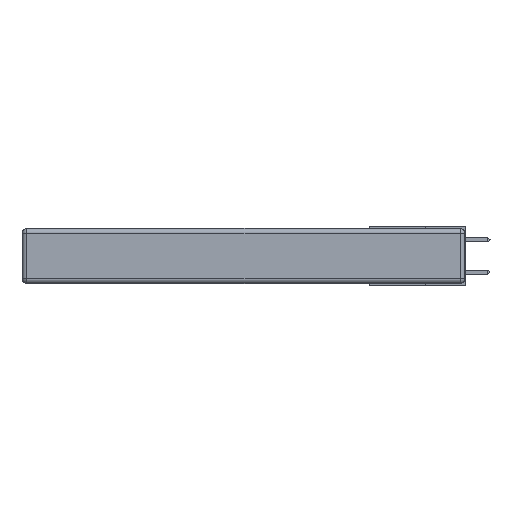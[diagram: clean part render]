
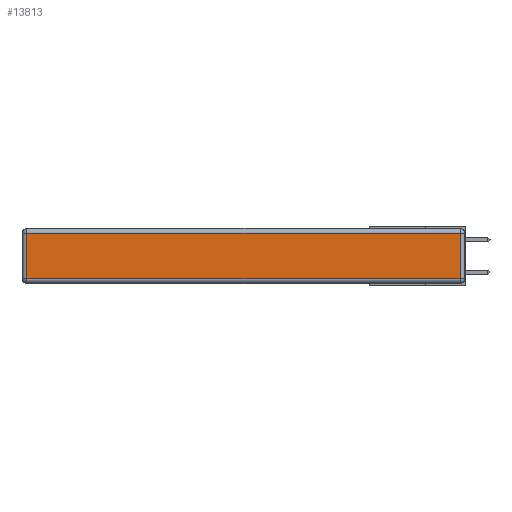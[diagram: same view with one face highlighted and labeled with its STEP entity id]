
A CAD part, left-side view. The second image highlights one B-rep face of the part: STEP entity #13813.
In plain terms, the highlighted planar face has unit normal (-1, 0, 0).
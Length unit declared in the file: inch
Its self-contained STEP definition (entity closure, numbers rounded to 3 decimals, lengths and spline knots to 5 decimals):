
#301 = DIRECTION ( 'NONE',  ( -1., 0., 0. ) ) ;
#597 = CARTESIAN_POINT ( 'NONE',  ( 0., 0., -0.313 ) ) ;
#2626 = FACE_OUTER_BOUND ( 'NONE', #26047, .T. ) ;
#2797 = VERTEX_POINT ( 'NONE', #15415 ) ;
#4282 = ORIENTED_EDGE ( 'NONE', *, *, #10737, .T. ) ;
#4748 = LINE ( 'NONE', #597, #14809 ) ;
#4893 = LINE ( 'NONE', #23380, #18332 ) ;
#6247 = CARTESIAN_POINT ( 'NONE',  ( 0., 2.75, -0.03 ) ) ;
#6422 = LINE ( 'NONE', #6247, #12806 ) ;
#7198 = VECTOR ( 'NONE', #26695, 39.37008 ) ;
#10737 = EDGE_CURVE ( 'NONE', #16903, #22494, #4748, .T. ) ;
#12715 = CARTESIAN_POINT ( 'NONE',  ( 0., 0.03, -0.313 ) ) ;
#12806 = VECTOR ( 'NONE', #23799, 39.37008 ) ;
#12847 = DIRECTION ( 'NONE',  ( 0., 0., -1. ) ) ;
#12964 = ORIENTED_EDGE ( 'NONE', *, *, #24188, .T. ) ;
#13006 = AXIS2_PLACEMENT_3D ( 'NONE', #24130, #301, #15243 ) ;
#13329 = PLANE ( 'NONE',  #13006 ) ;
#13633 = CARTESIAN_POINT ( 'NONE',  ( 0., 0.03, -0.343 ) ) ;
#13813 = ADVANCED_FACE ( 'NONE', ( #2626 ), #13329, .T. ) ;
#14432 = EDGE_CURVE ( 'NONE', #22494, #2797, #21616, .T. ) ;
#14809 = VECTOR ( 'NONE', #15531, 39.37008 ) ;
#14888 = CARTESIAN_POINT ( 'NONE',  ( 0., 2.72, -0.03 ) ) ;
#15243 = DIRECTION ( 'NONE',  ( 0., 0., 1. ) ) ;
#15415 = CARTESIAN_POINT ( 'NONE',  ( 0., 0.03, -0.03 ) ) ;
#15531 = DIRECTION ( 'NONE',  ( 0., -1., 0. ) ) ;
#16903 = VERTEX_POINT ( 'NONE', #18792 ) ;
#17005 = VERTEX_POINT ( 'NONE', #14888 ) ;
#18332 = VECTOR ( 'NONE', #12847, 39.37008 ) ;
#18792 = CARTESIAN_POINT ( 'NONE',  ( 0., 2.72, -0.313 ) ) ;
#19615 = EDGE_CURVE ( 'NONE', #17005, #16903, #4893, .T. ) ;
#21616 = LINE ( 'NONE', #13633, #7198 ) ;
#22494 = VERTEX_POINT ( 'NONE', #12715 ) ;
#23380 = CARTESIAN_POINT ( 'NONE',  ( 0., 2.72, -0.343 ) ) ;
#23799 = DIRECTION ( 'NONE',  ( 0., 1., 0. ) ) ;
#24026 = ORIENTED_EDGE ( 'NONE', *, *, #19615, .T. ) ;
#24130 = CARTESIAN_POINT ( 'NONE',  ( 0., 0., -0.343 ) ) ;
#24188 = EDGE_CURVE ( 'NONE', #2797, #17005, #6422, .T. ) ;
#24922 = ORIENTED_EDGE ( 'NONE', *, *, #14432, .T. ) ;
#26047 = EDGE_LOOP ( 'NONE', ( #4282, #24922, #12964, #24026 ) ) ;
#26695 = DIRECTION ( 'NONE',  ( 0., 0., 1. ) ) ;
